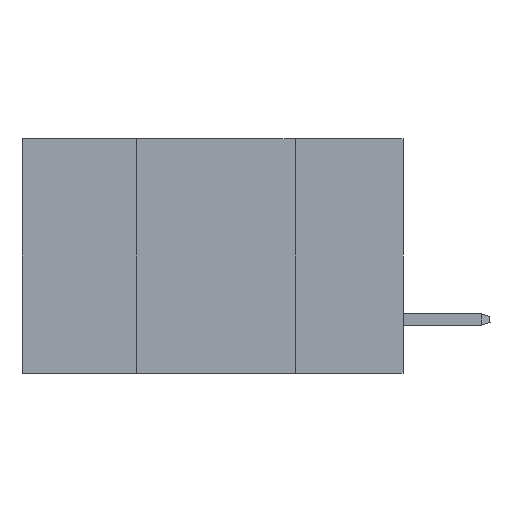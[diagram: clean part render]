
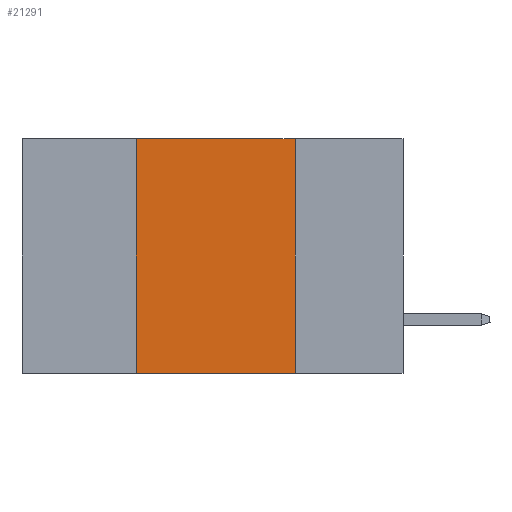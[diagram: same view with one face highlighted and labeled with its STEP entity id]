
A CAD part, left-side view. The second image highlights one B-rep face of the part: STEP entity #21291.
In plain terms, the highlighted planar face has unit normal (-1, 0, 0).
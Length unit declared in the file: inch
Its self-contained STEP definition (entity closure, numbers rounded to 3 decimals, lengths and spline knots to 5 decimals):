
#683 = EDGE_CURVE ( 'NONE', #2999, #23144, #22152, .T. ) ;
#1052 = CARTESIAN_POINT ( 'NONE',  ( 0., 0.17, 0. ) ) ;
#2004 = LINE ( 'NONE', #9173, #8101 ) ;
#2842 = VECTOR ( 'NONE', #24568, 39.37008 ) ;
#2940 = VERTEX_POINT ( 'NONE', #27300 ) ;
#2999 = VERTEX_POINT ( 'NONE', #9464 ) ;
#3617 = ORIENTED_EDGE ( 'NONE', *, *, #26033, .F. ) ;
#7988 = EDGE_CURVE ( 'NONE', #23144, #15764, #19520, .T. ) ;
#8101 = VECTOR ( 'NONE', #20385, 39.37008 ) ;
#8821 = CARTESIAN_POINT ( 'NONE',  ( 0., 0.6, 0. ) ) ;
#9173 = CARTESIAN_POINT ( 'NONE',  ( 0., 0.6, -0.37 ) ) ;
#9464 = CARTESIAN_POINT ( 'NONE',  ( 0., 0.42, -0.37 ) ) ;
#10344 = DIRECTION ( 'NONE',  ( 0., 0., -1. ) ) ;
#10553 = EDGE_CURVE ( 'NONE', #2999, #2940, #2004, .T. ) ;
#11289 = ORIENTED_EDGE ( 'NONE', *, *, #683, .F. ) ;
#12692 = VECTOR ( 'NONE', #10344, 39.37008 ) ;
#13001 = DIRECTION ( 'NONE',  ( 0., -1., 0. ) ) ;
#13520 = DIRECTION ( 'NONE',  ( 0., 0., -1. ) ) ;
#13674 = FACE_OUTER_BOUND ( 'NONE', #18162, .T. ) ;
#14547 = ORIENTED_EDGE ( 'NONE', *, *, #7988, .F. ) ;
#15764 = VERTEX_POINT ( 'NONE', #27617 ) ;
#16864 = ORIENTED_EDGE ( 'NONE', *, *, #10553, .T. ) ;
#17594 = CARTESIAN_POINT ( 'NONE',  ( 0., 0.42, 0. ) ) ;
#18162 = EDGE_LOOP ( 'NONE', ( #3617, #14547, #11289, #16864 ) ) ;
#18953 = LINE ( 'NONE', #1052, #12692 ) ;
#19520 = LINE ( 'NONE', #24203, #24017 ) ;
#20385 = DIRECTION ( 'NONE',  ( 0., -1., 0. ) ) ;
#20639 = PLANE ( 'NONE',  #28397 ) ;
#21291 = ADVANCED_FACE ( 'NONE', ( #13674 ), #20639, .F. ) ;
#21449 = CARTESIAN_POINT ( 'NONE',  ( 0., 0.42, 0. ) ) ;
#22152 = LINE ( 'NONE', #17594, #2842 ) ;
#23144 = VERTEX_POINT ( 'NONE', #21449 ) ;
#24017 = VECTOR ( 'NONE', #13001, 39.37008 ) ;
#24203 = CARTESIAN_POINT ( 'NONE',  ( 0., 0.6, 0. ) ) ;
#24568 = DIRECTION ( 'NONE',  ( 0., 0., 1. ) ) ;
#26033 = EDGE_CURVE ( 'NONE', #15764, #2940, #18953, .T. ) ;
#27300 = CARTESIAN_POINT ( 'NONE',  ( 0., 0.17, -0.37 ) ) ;
#27617 = CARTESIAN_POINT ( 'NONE',  ( 0., 0.17, 0. ) ) ;
#28397 = AXIS2_PLACEMENT_3D ( 'NONE', #8821, #29396, #13520 ) ;
#29396 = DIRECTION ( 'NONE',  ( 1., 0., 0. ) ) ;
